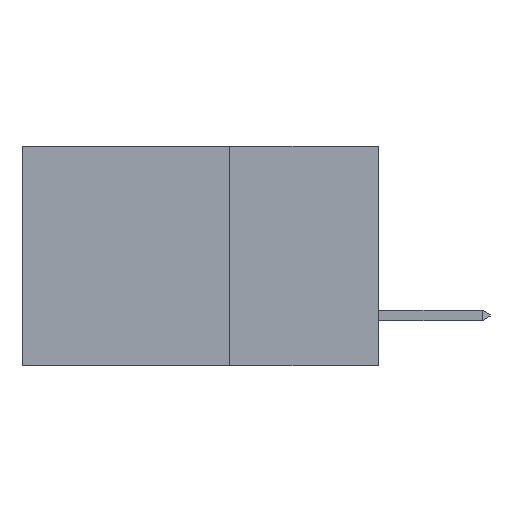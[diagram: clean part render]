
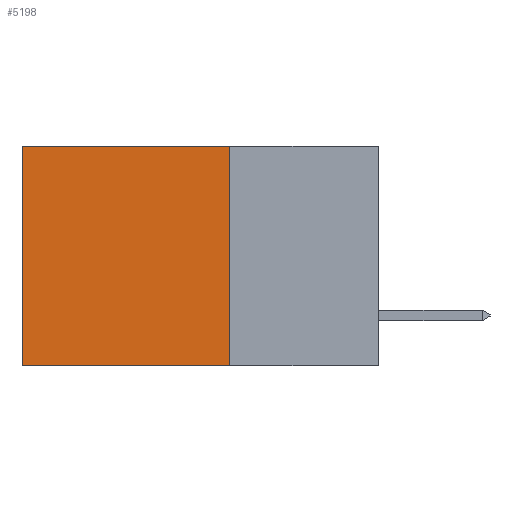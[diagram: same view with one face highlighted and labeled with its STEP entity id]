
A CAD part, left-side view. The second image highlights one B-rep face of the part: STEP entity #5198.
In plain terms, the highlighted planar face has unit normal (-1, 0, 0).
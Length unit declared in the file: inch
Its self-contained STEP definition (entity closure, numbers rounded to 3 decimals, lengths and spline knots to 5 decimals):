
#169 = VERTEX_POINT ( 'NONE', #10620 ) ;
#592 = VECTOR ( 'NONE', #9462, 39.37008 ) ;
#853 = ORIENTED_EDGE ( 'NONE', *, *, #12830, .F. ) ;
#903 = DIRECTION ( 'NONE',  ( 0., 0., -1. ) ) ;
#2816 = VECTOR ( 'NONE', #16911, 39.37008 ) ;
#3637 = CARTESIAN_POINT ( 'NONE',  ( 0.298, 0.6, 0. ) ) ;
#5198 = ADVANCED_FACE ( 'NONE', ( #10160 ), #14716, .F. ) ;
#6346 = EDGE_CURVE ( 'NONE', #11329, #10874, #21447, .T. ) ;
#6436 = ORIENTED_EDGE ( 'NONE', *, *, #6346, .F. ) ;
#7339 = LINE ( 'NONE', #15684, #20699 ) ;
#8468 = VECTOR ( 'NONE', #13775, 39.37008 ) ;
#9462 = DIRECTION ( 'NONE',  ( 0., 1., 0. ) ) ;
#10105 = LINE ( 'NONE', #19852, #592 ) ;
#10160 = FACE_OUTER_BOUND ( 'NONE', #21833, .T. ) ;
#10182 = AXIS2_PLACEMENT_3D ( 'NONE', #17972, #16568, #903 ) ;
#10254 = CARTESIAN_POINT ( 'NONE',  ( 0.298, 0.6, 0. ) ) ;
#10620 = CARTESIAN_POINT ( 'NONE',  ( 0.298, 0.6, -0.37 ) ) ;
#10874 = VERTEX_POINT ( 'NONE', #11674 ) ;
#11329 = VERTEX_POINT ( 'NONE', #18608 ) ;
#11674 = CARTESIAN_POINT ( 'NONE',  ( 0.298, 0.25, -0.37 ) ) ;
#12774 = EDGE_CURVE ( 'NONE', #16030, #169, #22289, .T. ) ;
#12830 = EDGE_CURVE ( 'NONE', #10874, #169, #7339, .T. ) ;
#12947 = ORIENTED_EDGE ( 'NONE', *, *, #12774, .T. ) ;
#13775 = DIRECTION ( 'NONE',  ( 0., 0., -1. ) ) ;
#14608 = EDGE_CURVE ( 'NONE', #11329, #16030, #10105, .T. ) ;
#14716 = PLANE ( 'NONE',  #10182 ) ;
#15153 = CARTESIAN_POINT ( 'NONE',  ( 0.298, 0.25, 0. ) ) ;
#15684 = CARTESIAN_POINT ( 'NONE',  ( 0.298, 0.25, -0.37 ) ) ;
#16030 = VERTEX_POINT ( 'NONE', #3637 ) ;
#16568 = DIRECTION ( 'NONE',  ( 1., 0., 0. ) ) ;
#16911 = DIRECTION ( 'NONE',  ( 0., 0., -1. ) ) ;
#17972 = CARTESIAN_POINT ( 'NONE',  ( 0.298, 0.25, 0. ) ) ;
#18608 = CARTESIAN_POINT ( 'NONE',  ( 0.298, 0.25, 0. ) ) ;
#19852 = CARTESIAN_POINT ( 'NONE',  ( 0.298, 0.25, 0. ) ) ;
#20699 = VECTOR ( 'NONE', #20815, 39.37008 ) ;
#20815 = DIRECTION ( 'NONE',  ( 0., 1., 0. ) ) ;
#21447 = LINE ( 'NONE', #15153, #2816 ) ;
#21833 = EDGE_LOOP ( 'NONE', ( #12947, #853, #6436, #22652 ) ) ;
#22289 = LINE ( 'NONE', #10254, #8468 ) ;
#22652 = ORIENTED_EDGE ( 'NONE', *, *, #14608, .T. ) ;
